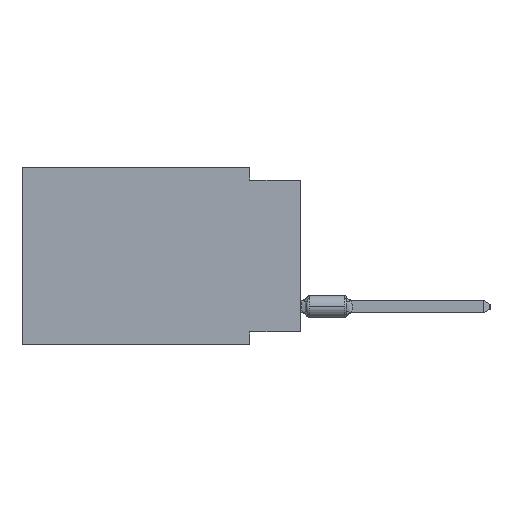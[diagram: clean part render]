
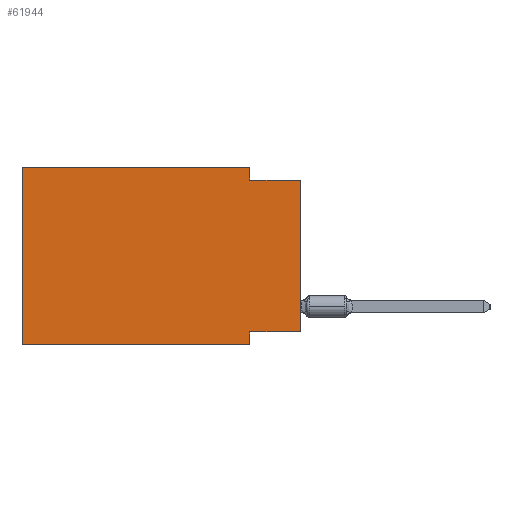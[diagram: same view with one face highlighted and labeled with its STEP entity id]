
A CAD part, left-side view. The second image highlights one B-rep face of the part: STEP entity #61944.
In plain terms, the highlighted planar face has unit normal (-1, 0, 0).
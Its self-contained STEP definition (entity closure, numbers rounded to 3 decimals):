
#718 = EDGE_LOOP ( 'NONE', ( #19546, #31141, #42625, #28116, #33074, #8544, #55862, #45845 ) ) ;
#4590 = LINE ( 'NONE', #47955, #39361 ) ;
#4811 = CARTESIAN_POINT ( 'NONE',  ( 0., 2.54, -8.89 ) ) ;
#5277 = VERTEX_POINT ( 'NONE', #63179 ) ;
#7072 = EDGE_CURVE ( 'NONE', #31820, #5277, #34517, .T. ) ;
#7325 = CARTESIAN_POINT ( 'NONE',  ( 0., 2.54, 0. ) ) ;
#8367 = EDGE_CURVE ( 'NONE', #31820, #28516, #59126, .T. ) ;
#8544 = ORIENTED_EDGE ( 'NONE', *, *, #8367, .T. ) ;
#9730 = DIRECTION ( 'NONE',  ( 0., 0., 1. ) ) ;
#10295 = VECTOR ( 'NONE', #57032, 1000. ) ;
#10650 = CARTESIAN_POINT ( 'NONE',  ( 0., 0., -0.635 ) ) ;
#11894 = DIRECTION ( 'NONE',  ( 1., 0., 0. ) ) ;
#13384 = DIRECTION ( 'NONE',  ( 0., -1., 0. ) ) ;
#13717 = CARTESIAN_POINT ( 'NONE',  ( 0., 2.54, 0. ) ) ;
#16458 = FACE_OUTER_BOUND ( 'NONE', #718, .T. ) ;
#16562 = VERTEX_POINT ( 'NONE', #10650 ) ;
#19148 = EDGE_CURVE ( 'NONE', #25439, #25642, #58940, .T. ) ;
#19546 = ORIENTED_EDGE ( 'NONE', *, *, #38652, .T. ) ;
#21866 = VECTOR ( 'NONE', #45660, 1000. ) ;
#22295 = DIRECTION ( 'NONE',  ( 0., 0., -1. ) ) ;
#24363 = DIRECTION ( 'NONE',  ( 0., 1., 0. ) ) ;
#25439 = VERTEX_POINT ( 'NONE', #55304 ) ;
#25642 = VERTEX_POINT ( 'NONE', #57678 ) ;
#26356 = CARTESIAN_POINT ( 'NONE',  ( 0., 2.54, -0.635 ) ) ;
#28116 = ORIENTED_EDGE ( 'NONE', *, *, #61573, .F. ) ;
#28516 = VERTEX_POINT ( 'NONE', #55690 ) ;
#28918 = VECTOR ( 'NONE', #22295, 1000. ) ;
#29353 = VERTEX_POINT ( 'NONE', #13717 ) ;
#31141 = ORIENTED_EDGE ( 'NONE', *, *, #44026, .F. ) ;
#31820 = VERTEX_POINT ( 'NONE', #35329 ) ;
#32087 = LINE ( 'NONE', #7325, #28918 ) ;
#32242 = LINE ( 'NONE', #42985, #58336 ) ;
#33074 = ORIENTED_EDGE ( 'NONE', *, *, #7072, .F. ) ;
#34517 = LINE ( 'NONE', #54396, #41479 ) ;
#35329 = CARTESIAN_POINT ( 'NONE',  ( 0., 13.97, -8.89 ) ) ;
#36360 = DIRECTION ( 'NONE',  ( 0., 0., -1. ) ) ;
#37280 = VERTEX_POINT ( 'NONE', #26356 ) ;
#38652 = EDGE_CURVE ( 'NONE', #25439, #16562, #32242, .T. ) ;
#39353 = LINE ( 'NONE', #4811, #63458 ) ;
#39361 = VECTOR ( 'NONE', #13384, 1000. ) ;
#40839 = VECTOR ( 'NONE', #24363, 1000. ) ;
#41266 = PLANE ( 'NONE',  #64516 ) ;
#41410 = LINE ( 'NONE', #52126, #10295 ) ;
#41479 = VECTOR ( 'NONE', #9730, 1000. ) ;
#42625 = ORIENTED_EDGE ( 'NONE', *, *, #60863, .F. ) ;
#42985 = CARTESIAN_POINT ( 'NONE',  ( 0., 0., 0. ) ) ;
#44026 = EDGE_CURVE ( 'NONE', #37280, #16562, #4590, .T. ) ;
#45660 = DIRECTION ( 'NONE',  ( 0., -1., 0. ) ) ;
#45845 = ORIENTED_EDGE ( 'NONE', *, *, #19148, .F. ) ;
#46129 = EDGE_CURVE ( 'NONE', #25642, #28516, #39353, .T. ) ;
#46145 = CARTESIAN_POINT ( 'NONE',  ( 0., 13.97, 0. ) ) ;
#47955 = CARTESIAN_POINT ( 'NONE',  ( 0., 0., -0.635 ) ) ;
#49485 = CARTESIAN_POINT ( 'NONE',  ( 0., 0., -8.255 ) ) ;
#49786 = DIRECTION ( 'NONE',  ( 0., 0., -1. ) ) ;
#52126 = CARTESIAN_POINT ( 'NONE',  ( 0., 13.97, 0. ) ) ;
#52447 = DIRECTION ( 'NONE',  ( 0., 0., 1. ) ) ;
#54396 = CARTESIAN_POINT ( 'NONE',  ( 0., 13.97, 0. ) ) ;
#55304 = CARTESIAN_POINT ( 'NONE',  ( 0., 0., -8.255 ) ) ;
#55690 = CARTESIAN_POINT ( 'NONE',  ( 0., 2.54, -8.89 ) ) ;
#55862 = ORIENTED_EDGE ( 'NONE', *, *, #46129, .F. ) ;
#57032 = DIRECTION ( 'NONE',  ( 0., -1., 0. ) ) ;
#57678 = CARTESIAN_POINT ( 'NONE',  ( 0., 2.54, -8.255 ) ) ;
#58336 = VECTOR ( 'NONE', #52447, 1000. ) ;
#58940 = LINE ( 'NONE', #49485, #40839 ) ;
#59126 = LINE ( 'NONE', #60662, #21866 ) ;
#60662 = CARTESIAN_POINT ( 'NONE',  ( 0., 13.97, -8.89 ) ) ;
#60863 = EDGE_CURVE ( 'NONE', #29353, #37280, #32087, .T. ) ;
#61573 = EDGE_CURVE ( 'NONE', #5277, #29353, #41410, .T. ) ;
#61944 = ADVANCED_FACE ( 'NONE', ( #16458 ), #41266, .F. ) ;
#63179 = CARTESIAN_POINT ( 'NONE',  ( 0., 13.97, 0. ) ) ;
#63458 = VECTOR ( 'NONE', #49786, 1000. ) ;
#64516 = AXIS2_PLACEMENT_3D ( 'NONE', #46145, #11894, #36360 ) ;
